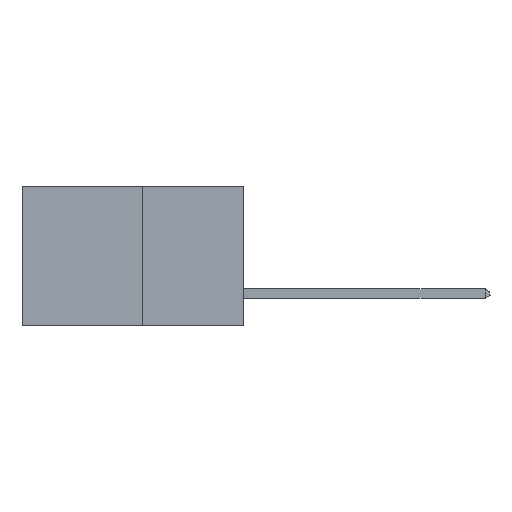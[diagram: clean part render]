
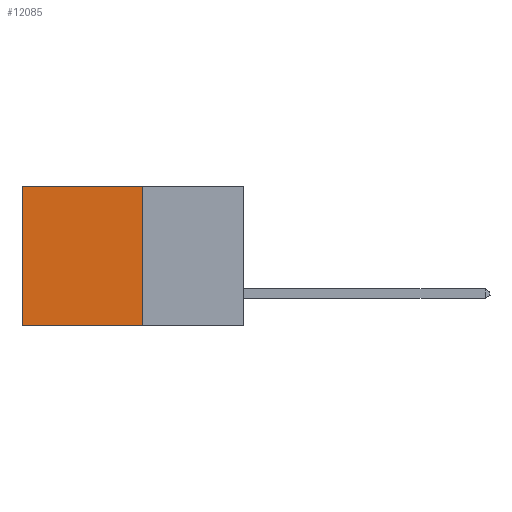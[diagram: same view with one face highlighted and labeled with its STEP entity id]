
A CAD part, left-side view. The second image highlights one B-rep face of the part: STEP entity #12085.
In plain terms, the highlighted planar face has unit normal (-1, 0, 0).
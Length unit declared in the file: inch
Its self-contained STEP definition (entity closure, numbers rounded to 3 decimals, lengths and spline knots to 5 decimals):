
#226 = VECTOR ( 'NONE', #8523, 39.37008 ) ;
#598 = CARTESIAN_POINT ( 'NONE',  ( 0.277, 0.27, 0. ) ) ;
#660 = DIRECTION ( 'NONE',  ( 1., 0., 0. ) ) ;
#730 = CARTESIAN_POINT ( 'NONE',  ( 0.277, 0.27, 0. ) ) ;
#1295 = AXIS2_PLACEMENT_3D ( 'NONE', #4922, #660, #10600 ) ;
#1584 = EDGE_CURVE ( 'NONE', #13650, #11546, #9226, .T. ) ;
#1959 = ORIENTED_EDGE ( 'NONE', *, *, #18080, .F. ) ;
#2565 = DIRECTION ( 'NONE',  ( 0., 0., -1. ) ) ;
#2603 = VECTOR ( 'NONE', #17724, 39.37008 ) ;
#3809 = CARTESIAN_POINT ( 'NONE',  ( 0.277, 0.59, -0.37 ) ) ;
#4078 = CARTESIAN_POINT ( 'NONE',  ( 0.277, 0.59, -0.37 ) ) ;
#4378 = EDGE_CURVE ( 'NONE', #16758, #11546, #4918, .T. ) ;
#4918 = LINE ( 'NONE', #4078, #16211 ) ;
#4922 = CARTESIAN_POINT ( 'NONE',  ( 0.277, 0.27, -0.37 ) ) ;
#6098 = ORIENTED_EDGE ( 'NONE', *, *, #1584, .F. ) ;
#6464 = EDGE_CURVE ( 'NONE', #9005, #16758, #6828, .T. ) ;
#6828 = LINE ( 'NONE', #730, #14389 ) ;
#8523 = DIRECTION ( 'NONE',  ( 0., 0., -1. ) ) ;
#9005 = VERTEX_POINT ( 'NONE', #598 ) ;
#9226 = LINE ( 'NONE', #11647, #2603 ) ;
#9476 = FACE_OUTER_BOUND ( 'NONE', #10569, .T. ) ;
#9698 = CARTESIAN_POINT ( 'NONE',  ( 0.277, 0.59, 0. ) ) ;
#10569 = EDGE_LOOP ( 'NONE', ( #12467, #6098, #1959, #13186 ) ) ;
#10600 = DIRECTION ( 'NONE',  ( 0., 0., -1. ) ) ;
#11546 = VERTEX_POINT ( 'NONE', #3809 ) ;
#11559 = LINE ( 'NONE', #17042, #226 ) ;
#11647 = CARTESIAN_POINT ( 'NONE',  ( 0.277, 0.27, -0.37 ) ) ;
#11955 = PLANE ( 'NONE',  #1295 ) ;
#12085 = ADVANCED_FACE ( 'NONE', ( #9476 ), #11955, .F. ) ;
#12467 = ORIENTED_EDGE ( 'NONE', *, *, #4378, .T. ) ;
#13186 = ORIENTED_EDGE ( 'NONE', *, *, #6464, .T. ) ;
#13214 = CARTESIAN_POINT ( 'NONE',  ( 0.277, 0.27, -0.37 ) ) ;
#13650 = VERTEX_POINT ( 'NONE', #13214 ) ;
#14389 = VECTOR ( 'NONE', #14925, 39.37008 ) ;
#14925 = DIRECTION ( 'NONE',  ( 0., 1., 0. ) ) ;
#16211 = VECTOR ( 'NONE', #2565, 39.37008 ) ;
#16758 = VERTEX_POINT ( 'NONE', #9698 ) ;
#17042 = CARTESIAN_POINT ( 'NONE',  ( 0.277, 0.27, -0.37 ) ) ;
#17724 = DIRECTION ( 'NONE',  ( 0., 1., 0. ) ) ;
#18080 = EDGE_CURVE ( 'NONE', #9005, #13650, #11559, .T. ) ;
